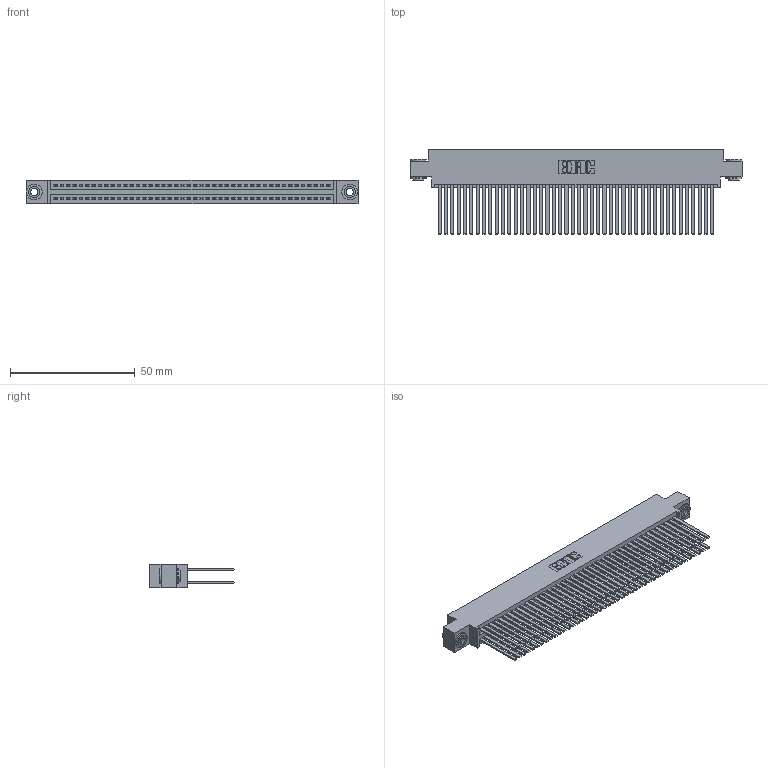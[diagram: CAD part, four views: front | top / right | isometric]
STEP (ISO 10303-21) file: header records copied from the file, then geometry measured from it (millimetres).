
FILE_DESCRIPTION (( 'STEP AP203' ), '1' );
FILE_NAME ('395-088-544-803.STEP', '2018-11-29T00:47:05', ( '' ), ( '' ), 'SwSTEP 2.0', 'SolidWorks 2016', '' );
FILE_SCHEMA (( 'CONFIG_CONTROL_DESIGN' ));
Length unit declared in the file: inch
Products named in the file (4): 345 Part_0.170 Offset - 0.156 Dia-TH; 395-088-544-803; 345-292-001_345-293-144; 345-250-002_345-250-002-102
Assembly tree (91 placements, depth 2):
  395-088-544-803
    345 Part_0.170 Offset - 0.156 Dia-TH
    345-292-001_345-293-144  x88
    345-250-002_345-250-002-102  x2
Bounding box: 132.97 x 33.96 x 9.4 mm (x, y, z)
Volume: 14074.9 mm3; surface area: 24807.8 mm2
Topology: 91 solids, 91 shells, 4040 faces, 11957 edges, 7850 vertices
Faces by surface type: plane 2646, cylinder 1386, cone 8
Entity records: 34852 total; most frequent: CARTESIAN_POINT 5815, ORIENTED_EDGE 5742, DIRECTION 5153, EDGE_CURVE 2871, LINE 2543, VECTOR 2543, VERTEX_POINT 1910, AXIS2_PLACEMENT_3D 1305
